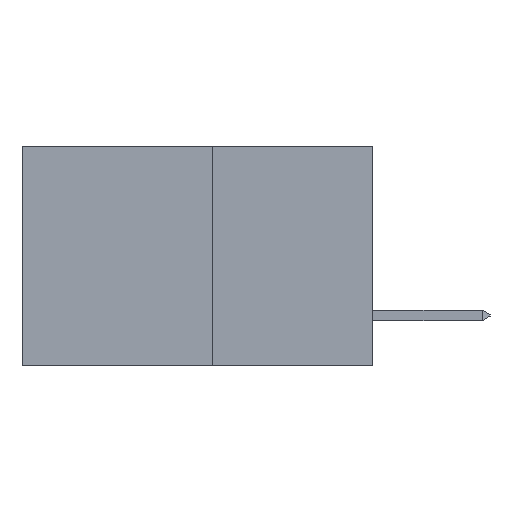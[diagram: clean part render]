
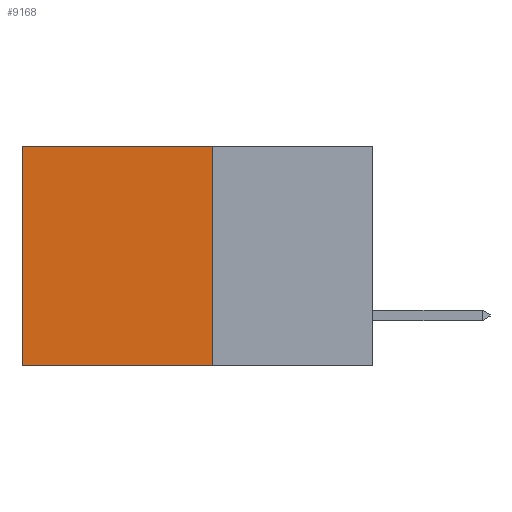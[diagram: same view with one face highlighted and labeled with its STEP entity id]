
A CAD part, left-side view. The second image highlights one B-rep face of the part: STEP entity #9168.
In plain terms, the highlighted planar face has unit normal (-1, 0, 0).
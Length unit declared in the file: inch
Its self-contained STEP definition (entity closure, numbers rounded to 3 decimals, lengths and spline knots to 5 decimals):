
#978 = EDGE_CURVE ( 'NONE', #8969, #3696, #3313, .T. ) ;
#1267 = FACE_OUTER_BOUND ( 'NONE', #7016, .T. ) ;
#1691 = LINE ( 'NONE', #7158, #12369 ) ;
#1992 = CARTESIAN_POINT ( 'NONE',  ( 0.277, 0.27, -0.37 ) ) ;
#2821 = LINE ( 'NONE', #10739, #5959 ) ;
#2987 = DIRECTION ( 'NONE',  ( 0., 0., -1. ) ) ;
#3112 = VERTEX_POINT ( 'NONE', #7212 ) ;
#3224 = ORIENTED_EDGE ( 'NONE', *, *, #13257, .F. ) ;
#3313 = LINE ( 'NONE', #8255, #11224 ) ;
#3557 = ORIENTED_EDGE ( 'NONE', *, *, #978, .T. ) ;
#3696 = VERTEX_POINT ( 'NONE', #11426 ) ;
#3698 = VERTEX_POINT ( 'NONE', #12046 ) ;
#4078 = ORIENTED_EDGE ( 'NONE', *, *, #12406, .T. ) ;
#4164 = VECTOR ( 'NONE', #11498, 39.37008 ) ;
#4354 = EDGE_CURVE ( 'NONE', #3698, #3112, #8374, .T. ) ;
#4894 = DIRECTION ( 'NONE',  ( 0., 1., 0. ) ) ;
#5200 = DIRECTION ( 'NONE',  ( 1., 0., 0. ) ) ;
#5941 = CARTESIAN_POINT ( 'NONE',  ( 0.277, 0.27, 0. ) ) ;
#5959 = VECTOR ( 'NONE', #11770, 39.37008 ) ;
#6431 = AXIS2_PLACEMENT_3D ( 'NONE', #1992, #5200, #12335 ) ;
#7016 = EDGE_LOOP ( 'NONE', ( #4078, #11145, #3224, #3557 ) ) ;
#7158 = CARTESIAN_POINT ( 'NONE',  ( 0.277, 0.59, -0.37 ) ) ;
#7212 = CARTESIAN_POINT ( 'NONE',  ( 0.277, 0.59, -0.37 ) ) ;
#8255 = CARTESIAN_POINT ( 'NONE',  ( 0.277, 0.27, 0. ) ) ;
#8374 = LINE ( 'NONE', #11518, #4164 ) ;
#8969 = VERTEX_POINT ( 'NONE', #5941 ) ;
#9168 = ADVANCED_FACE ( 'NONE', ( #1267 ), #11361, .F. ) ;
#10739 = CARTESIAN_POINT ( 'NONE',  ( 0.277, 0.27, -0.37 ) ) ;
#11145 = ORIENTED_EDGE ( 'NONE', *, *, #4354, .F. ) ;
#11224 = VECTOR ( 'NONE', #4894, 39.37008 ) ;
#11361 = PLANE ( 'NONE',  #6431 ) ;
#11426 = CARTESIAN_POINT ( 'NONE',  ( 0.277, 0.59, 0. ) ) ;
#11498 = DIRECTION ( 'NONE',  ( 0., 1., 0. ) ) ;
#11518 = CARTESIAN_POINT ( 'NONE',  ( 0.277, 0.27, -0.37 ) ) ;
#11770 = DIRECTION ( 'NONE',  ( 0., 0., -1. ) ) ;
#12046 = CARTESIAN_POINT ( 'NONE',  ( 0.277, 0.27, -0.37 ) ) ;
#12335 = DIRECTION ( 'NONE',  ( 0., 0., -1. ) ) ;
#12369 = VECTOR ( 'NONE', #2987, 39.37008 ) ;
#12406 = EDGE_CURVE ( 'NONE', #3696, #3112, #1691, .T. ) ;
#13257 = EDGE_CURVE ( 'NONE', #8969, #3698, #2821, .T. ) ;
